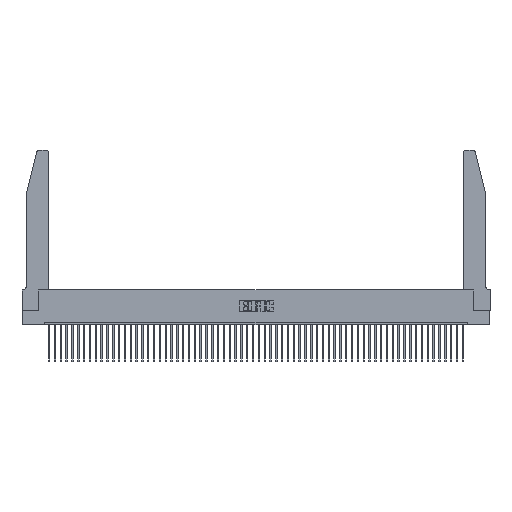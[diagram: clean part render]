
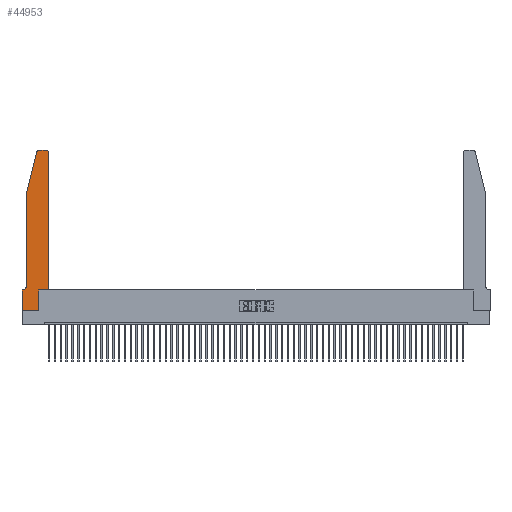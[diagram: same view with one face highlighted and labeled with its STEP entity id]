
A CAD part, top view. The second image highlights one B-rep face of the part: STEP entity #44953.
In plain terms, the highlighted planar face has unit normal (0, 0, 1).
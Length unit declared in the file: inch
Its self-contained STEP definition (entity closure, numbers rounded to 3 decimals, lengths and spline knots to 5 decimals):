
#292 = VERTEX_POINT ( 'NONE', #22463 ) ;
#1158 = EDGE_CURVE ( 'NONE', #13838, #29640, #31435, .T. ) ;
#1229 = EDGE_CURVE ( 'NONE', #292, #40355, #4788, .T. ) ;
#2292 = DIRECTION ( 'NONE',  ( 1., 0., 0. ) ) ;
#2351 = ORIENTED_EDGE ( 'NONE', *, *, #4294, .T. ) ;
#3685 = CARTESIAN_POINT ( 'NONE',  ( 0.2605, 2.75, 0.37 ) ) ;
#4294 = EDGE_CURVE ( 'NONE', #29640, #29583, #20560, .T. ) ;
#4599 = ORIENTED_EDGE ( 'NONE', *, *, #6364, .T. ) ;
#4788 = LINE ( 'NONE', #26230, #30043 ) ;
#5172 = VERTEX_POINT ( 'NONE', #27643 ) ;
#6299 = DIRECTION ( 'NONE',  ( -1., 0., 0. ) ) ;
#6364 = EDGE_CURVE ( 'NONE', #37228, #40752, #30144, .T. ) ;
#6368 = ORIENTED_EDGE ( 'NONE', *, *, #1158, .T. ) ;
#6424 = CARTESIAN_POINT ( 'NONE',  ( 0.2865, 0.35, 0.37 ) ) ;
#7796 = DIRECTION ( 'NONE',  ( 1., 0., 0. ) ) ;
#7850 = FACE_OUTER_BOUND ( 'NONE', #15400, .T. ) ;
#7922 = CARTESIAN_POINT ( 'NONE',  ( 0., 0., 0.37 ) ) ;
#9001 = EDGE_CURVE ( 'NONE', #40752, #5172, #10796, .T. ) ;
#9986 = EDGE_CURVE ( 'NONE', #48039, #36191, #30542, .T. ) ;
#10796 = CIRCLE ( 'NONE', #32984, 0.03 ) ;
#12082 = VECTOR ( 'NONE', #29316, 39.37008 ) ;
#12413 = VECTOR ( 'NONE', #41460, 39.37008 ) ;
#13360 = ORIENTED_EDGE ( 'NONE', *, *, #32408, .T. ) ;
#13373 = ORIENTED_EDGE ( 'NONE', *, *, #15092, .T. ) ;
#13838 = VERTEX_POINT ( 'NONE', #43435 ) ;
#14216 = ORIENTED_EDGE ( 'NONE', *, *, #9001, .T. ) ;
#15092 = EDGE_CURVE ( 'NONE', #24715, #37228, #15901, .T. ) ;
#15400 = EDGE_LOOP ( 'NONE', ( #4599, #14216, #44289, #6368, #2351, #25723, #29413, #13360, #17729, #35166, #22039, #13373 ) ) ;
#15841 = VECTOR ( 'NONE', #16097, 39.37008 ) ;
#15901 = CIRCLE ( 'NONE', #28467, 0.03 ) ;
#16097 = DIRECTION ( 'NONE',  ( -1., 0., 0. ) ) ;
#16186 = PLANE ( 'NONE',  #38562 ) ;
#17504 = CARTESIAN_POINT ( 'NONE',  ( 0.4205, 2.75, 0.37 ) ) ;
#17729 = ORIENTED_EDGE ( 'NONE', *, *, #30022, .T. ) ;
#20560 = CIRCLE ( 'NONE', #35996, 0.07 ) ;
#20802 = CARTESIAN_POINT ( 'NONE',  ( 0.4505, 0.35, 0.37 ) ) ;
#21536 = VECTOR ( 'NONE', #49465, 39.37008 ) ;
#22039 = ORIENTED_EDGE ( 'NONE', *, *, #27369, .T. ) ;
#22463 = CARTESIAN_POINT ( 'NONE',  ( 0., 0.35, 0.37 ) ) ;
#23834 = CARTESIAN_POINT ( 'NONE',  ( 0.0755, 2., 0.37 ) ) ;
#23904 = CARTESIAN_POINT ( 'NONE',  ( 0.0755, 2., 0.37 ) ) ;
#24414 = CARTESIAN_POINT ( 'NONE',  ( 0.4505, 0.35, 0.37 ) ) ;
#24514 = VECTOR ( 'NONE', #36668, 39.37008 ) ;
#24715 = VERTEX_POINT ( 'NONE', #45180 ) ;
#24919 = DIRECTION ( 'NONE',  ( 0., 1., 0. ) ) ;
#25723 = ORIENTED_EDGE ( 'NONE', *, *, #32421, .T. ) ;
#26230 = CARTESIAN_POINT ( 'NONE',  ( 0., 0., 0.37 ) ) ;
#26797 = CARTESIAN_POINT ( 'NONE',  ( 0.4205, 2.72, 0.37 ) ) ;
#27369 = EDGE_CURVE ( 'NONE', #36191, #24715, #46254, .T. ) ;
#27643 = CARTESIAN_POINT ( 'NONE',  ( 0.25487, 2.72718, 0.37 ) ) ;
#27766 = DIRECTION ( 'NONE',  ( 0., 0., 1. ) ) ;
#28467 = AXIS2_PLACEMENT_3D ( 'NONE', #26797, #48096, #44799 ) ;
#29316 = DIRECTION ( 'NONE',  ( 1., 0., 0. ) ) ;
#29413 = ORIENTED_EDGE ( 'NONE', *, *, #1229, .T. ) ;
#29583 = VERTEX_POINT ( 'NONE', #52722 ) ;
#29640 = VERTEX_POINT ( 'NONE', #39607 ) ;
#30022 = EDGE_CURVE ( 'NONE', #50859, #48039, #38042, .T. ) ;
#30043 = VECTOR ( 'NONE', #46865, 39.37008 ) ;
#30144 = LINE ( 'NONE', #3685, #41485 ) ;
#30542 = LINE ( 'NONE', #20802, #12082 ) ;
#31435 = LINE ( 'NONE', #23904, #21536 ) ;
#31699 = LINE ( 'NONE', #41462, #15841 ) ;
#32408 = EDGE_CURVE ( 'NONE', #40355, #50859, #34968, .T. ) ;
#32421 = EDGE_CURVE ( 'NONE', #29583, #292, #31699, .T. ) ;
#32984 = AXIS2_PLACEMENT_3D ( 'NONE', #44585, #27766, #2292 ) ;
#33187 = CARTESIAN_POINT ( 'NONE',  ( 0., 0., 0.37 ) ) ;
#34968 = LINE ( 'NONE', #33187, #24514 ) ;
#35166 = ORIENTED_EDGE ( 'NONE', *, *, #9986, .T. ) ;
#35372 = CARTESIAN_POINT ( 'NONE',  ( 0.4505, 0.35, 0.37 ) ) ;
#35836 = VECTOR ( 'NONE', #40666, 39.37008 ) ;
#35996 = AXIS2_PLACEMENT_3D ( 'NONE', #40394, #53551, #6299 ) ;
#36191 = VERTEX_POINT ( 'NONE', #35372 ) ;
#36668 = DIRECTION ( 'NONE',  ( 1., 0., 0. ) ) ;
#37228 = VERTEX_POINT ( 'NONE', #17504 ) ;
#37288 = CARTESIAN_POINT ( 'NONE',  ( 0., 0.35, 0.37 ) ) ;
#38042 = LINE ( 'NONE', #50639, #49954 ) ;
#38562 = AXIS2_PLACEMENT_3D ( 'NONE', #37288, #45452, #7796 ) ;
#39607 = CARTESIAN_POINT ( 'NONE',  ( 0.0755, 0.42, 0.37 ) ) ;
#40355 = VERTEX_POINT ( 'NONE', #7922 ) ;
#40394 = CARTESIAN_POINT ( 'NONE',  ( 0.0055, 0.42, 0.37 ) ) ;
#40666 = DIRECTION ( 'NONE',  ( -0.239, -0.971, 0. ) ) ;
#40752 = VERTEX_POINT ( 'NONE', #53859 ) ;
#41460 = DIRECTION ( 'NONE',  ( 0., 1., 0. ) ) ;
#41462 = CARTESIAN_POINT ( 'NONE',  ( 0.0755, 0.35, 0.37 ) ) ;
#41485 = VECTOR ( 'NONE', #54815, 39.37008 ) ;
#42556 = LINE ( 'NONE', #23834, #35836 ) ;
#43435 = CARTESIAN_POINT ( 'NONE',  ( 0.0755, 2., 0.37 ) ) ;
#44289 = ORIENTED_EDGE ( 'NONE', *, *, #49105, .T. ) ;
#44585 = CARTESIAN_POINT ( 'NONE',  ( 0.284, 2.72, 0.37 ) ) ;
#44799 = DIRECTION ( 'NONE',  ( 1., 0., 0. ) ) ;
#44938 = CARTESIAN_POINT ( 'NONE',  ( 0.2865, 0., 0.37 ) ) ;
#44953 = ADVANCED_FACE ( 'NONE', ( #7850 ), #16186, .T. ) ;
#45180 = CARTESIAN_POINT ( 'NONE',  ( 0.4505, 2.72, 0.37 ) ) ;
#45452 = DIRECTION ( 'NONE',  ( 0., 0., 1. ) ) ;
#46254 = LINE ( 'NONE', #24414, #12413 ) ;
#46865 = DIRECTION ( 'NONE',  ( 0., -1., 0. ) ) ;
#48039 = VERTEX_POINT ( 'NONE', #6424 ) ;
#48096 = DIRECTION ( 'NONE',  ( 0., 0., 1. ) ) ;
#49105 = EDGE_CURVE ( 'NONE', #5172, #13838, #42556, .T. ) ;
#49465 = DIRECTION ( 'NONE',  ( 0., -1., 0. ) ) ;
#49954 = VECTOR ( 'NONE', #24919, 39.37008 ) ;
#50639 = CARTESIAN_POINT ( 'NONE',  ( 0.2865, 0.35, 0.37 ) ) ;
#50859 = VERTEX_POINT ( 'NONE', #44938 ) ;
#52722 = CARTESIAN_POINT ( 'NONE',  ( 0.0055, 0.35, 0.37 ) ) ;
#53551 = DIRECTION ( 'NONE',  ( 0., 0., -1. ) ) ;
#53859 = CARTESIAN_POINT ( 'NONE',  ( 0.284, 2.75, 0.37 ) ) ;
#54815 = DIRECTION ( 'NONE',  ( -1., 0., 0. ) ) ;
